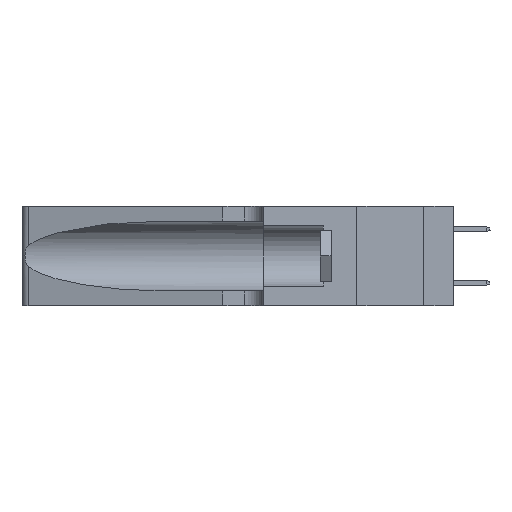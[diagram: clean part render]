
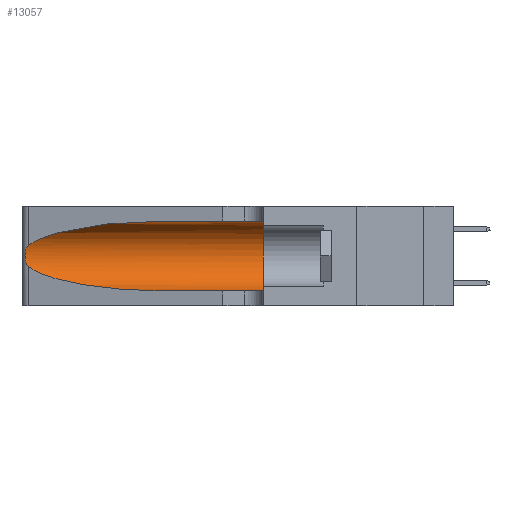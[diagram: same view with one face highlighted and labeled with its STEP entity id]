
A CAD part, left-side view. The second image highlights one B-rep face of the part: STEP entity #13057.
In plain terms, the highlighted cylindrical face has radius 3.308 mm (diameter 6.617 mm), a partial arc.
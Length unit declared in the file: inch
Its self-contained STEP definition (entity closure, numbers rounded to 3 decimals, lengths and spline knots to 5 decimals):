
#863 = ORIENTED_EDGE ( 'NONE', *, *, #18029, .T. ) ;
#1725 = DIRECTION ( 'NONE',  ( 0., 1., 0. ) ) ;
#1914 = CARTESIAN_POINT ( 'NONE',  ( 0.25856, 1.23593, 0.16098 ) ) ;
#2134 = CARTESIAN_POINT ( 'NONE',  ( 0.25555, 1.22994, 0.2215 ) ) ;
#2433 = EDGE_CURVE ( 'NONE', #37462, #30341, #22321, .T. ) ;
#3143 = VERTEX_POINT ( 'NONE', #30191 ) ;
#4962 = AXIS2_PLACEMENT_3D ( 'NONE', #8616, #1725, #5499 ) ;
#5132 = DIRECTION ( 'NONE',  ( 0., 0., -1. ) ) ;
#5239 = CARTESIAN_POINT ( 'NONE',  ( 0.26075, 1.23896, 0.178 ) ) ;
#5499 = DIRECTION ( 'NONE',  ( 0., 0., 1. ) ) ;
#6105 = DIRECTION ( 'NONE',  ( 0., -1., 0. ) ) ;
#6363 = EDGE_CURVE ( 'NONE', #30341, #28219, #10598, .T. ) ;
#8273 = EDGE_CURVE ( 'NONE', #3143, #10191, #37781, .T. ) ;
#8577 = CARTESIAN_POINT ( 'NONE',  ( 0.26018, 1.23835, 0.19895 ) ) ;
#8616 = CARTESIAN_POINT ( 'NONE',  ( 0.1305, 0.35, 0.185 ) ) ;
#9137 = ORIENTED_EDGE ( 'NONE', *, *, #8273, .T. ) ;
#10191 = VERTEX_POINT ( 'NONE', #12703 ) ;
#10598 = CIRCLE ( 'NONE', #4962, 0.13025 ) ;
#10744 = ORIENTED_EDGE ( 'NONE', *, *, #6363, .F. ) ;
#10781 = CARTESIAN_POINT ( 'NONE',  ( 0.18966, 0.96281, 0.31525 ) ) ;
#11106 = FACE_OUTER_BOUND ( 'NONE', #35113, .T. ) ;
#11331 = CYLINDRICAL_SURFACE ( 'NONE', #17786, 0.13025 ) ;
#11534 = CARTESIAN_POINT ( 'NONE',  ( 0.25487, 1.22718, 0.14631 ) ) ;
#12703 = CARTESIAN_POINT ( 'NONE',  ( 0.25487, 1.22718, 0.14631 ) ) ;
#13057 = ADVANCED_FACE ( 'NONE', ( #11106 ), #11331, .F. ) ;
#13968 = CARTESIAN_POINT ( 'NONE',  ( 0.2373, 1.15595, 0.08982 ) ) ;
#14073 = CARTESIAN_POINT ( 'NONE',  ( 0.1305, 0.72297, 0.31525 ) ) ;
#15653 = CARTESIAN_POINT ( 'NONE',  ( 0.25854, 1.2359, 0.20912 ) ) ;
#16092 = CARTESIAN_POINT ( 'NONE',  ( 0.1305, 1.61858, 0.05475 ) ) ;
#16347 = VECTOR ( 'NONE', #6105, 39.37008 ) ;
#17304 =( BOUNDED_CURVE ( )  B_SPLINE_CURVE ( 3, ( #41151, #10781, #40265, #23463 ),
 .UNSPECIFIED., .F., .T. ) 
 B_SPLINE_CURVE_WITH_KNOTS ( ( 4, 4 ),
 ( 1.5708, 2.84003 ),
 .UNSPECIFIED. ) 
 CURVE ( )  GEOMETRIC_REPRESENTATION_ITEM ( )  RATIONAL_B_SPLINE_CURVE ( ( 1., 0.87, 0.87, 1. ) ) 
 REPRESENTATION_ITEM ( '' )  );
#17517 = CARTESIAN_POINT ( 'NONE',  ( 0.1305, 0.72297, 0.05475 ) ) ;
#17786 = AXIS2_PLACEMENT_3D ( 'NONE', #25350, #35471, #5132 ) ;
#18029 = EDGE_CURVE ( 'NONE', #37462, #3143, #17304, .T. ) ;
#18058 = ORIENTED_EDGE ( 'NONE', *, *, #42897, .T. ) ;
#19828 = CARTESIAN_POINT ( 'NONE',  ( 0.25555, 1.22993, 0.14849 ) ) ;
#22021 = VERTEX_POINT ( 'NONE', #35076 ) ;
#22321 = LINE ( 'NONE', #32707, #16347 ) ;
#22568 = DIRECTION ( 'NONE',  ( 0., -1., 0. ) ) ;
#23463 = CARTESIAN_POINT ( 'NONE',  ( 0.25487, 1.22718, 0.22369 ) ) ;
#24613 = ORIENTED_EDGE ( 'NONE', *, *, #37897, .T. ) ;
#25350 = CARTESIAN_POINT ( 'NONE',  ( 0.1305, 1.61858, 0.185 ) ) ;
#25459 = CARTESIAN_POINT ( 'NONE',  ( 0.25639, 1.23184, 0.21858 ) ) ;
#27272 = CARTESIAN_POINT ( 'NONE',  ( 0.1305, 0.35, 0.31525 ) ) ;
#28219 = VERTEX_POINT ( 'NONE', #38660 ) ;
#29186 = CARTESIAN_POINT ( 'NONE',  ( 0.26075, 1.23896, 0.19203 ) ) ;
#30023 = CARTESIAN_POINT ( 'NONE',  ( 0.25487, 1.22718, 0.14631 ) ) ;
#30191 = CARTESIAN_POINT ( 'NONE',  ( 0.25487, 1.22718, 0.22369 ) ) ;
#30242 = CARTESIAN_POINT ( 'NONE',  ( 0.25639, 1.23186, 0.15144 ) ) ;
#30341 = VERTEX_POINT ( 'NONE', #27272 ) ;
#30825 = CARTESIAN_POINT ( 'NONE',  ( 0.18966, 0.96281, 0.05475 ) ) ;
#32271 = CARTESIAN_POINT ( 'NONE',  ( 0.26017, 1.23833, 0.17102 ) ) ;
#32707 = CARTESIAN_POINT ( 'NONE',  ( 0.1305, 1.61858, 0.31525 ) ) ;
#32940 = LINE ( 'NONE', #16092, #36297 ) ;
#35076 = CARTESIAN_POINT ( 'NONE',  ( 0.1305, 0.72297, 0.05475 ) ) ;
#35113 = EDGE_LOOP ( 'NONE', ( #863, #9137, #24613, #18058, #10744, #40123 ) ) ;
#35471 = DIRECTION ( 'NONE',  ( 0., -1., 0. ) ) ;
#35581 = CARTESIAN_POINT ( 'NONE',  ( 0.25487, 1.22718, 0.22369 ) ) ;
#35684 =( BOUNDED_CURVE ( )  B_SPLINE_CURVE ( 3, ( #11534, #13968, #30825, #17517 ),
 .UNSPECIFIED., .F., .T. ) 
 B_SPLINE_CURVE_WITH_KNOTS ( ( 4, 4 ),
 ( 3.44316, 4.71239 ),
 .UNSPECIFIED. ) 
 CURVE ( )  GEOMETRIC_REPRESENTATION_ITEM ( )  RATIONAL_B_SPLINE_CURVE ( ( 1., 0.87, 0.87, 1. ) ) 
 REPRESENTATION_ITEM ( '' )  );
#36297 = VECTOR ( 'NONE', #22568, 39.37008 ) ;
#37462 = VERTEX_POINT ( 'NONE', #14073 ) ;
#37781 = B_SPLINE_CURVE_WITH_KNOTS ( 'NONE', 3,
 ( #35581, #2134, #25459, #38939, #15653, #8577, #29186, #5239, #32271, #1914, #41804, #30242, #19828, #30023 ),
 .UNSPECIFIED., .F., .F.,
 ( 4, 2, 2, 2, 2, 2, 4 ),
 ( 0., 0.00027, 0.00053, 0.00107, 0.0016, 0.00187, 0.00214 ),
 .UNSPECIFIED. ) ;
#37897 = EDGE_CURVE ( 'NONE', #10191, #22021, #35684, .T. ) ;
#38660 = CARTESIAN_POINT ( 'NONE',  ( 0.1305, 0.35, 0.05475 ) ) ;
#38939 = CARTESIAN_POINT ( 'NONE',  ( 0.25787, 1.23484, 0.2124 ) ) ;
#40123 = ORIENTED_EDGE ( 'NONE', *, *, #2433, .F. ) ;
#40265 = CARTESIAN_POINT ( 'NONE',  ( 0.2373, 1.15595, 0.28018 ) ) ;
#41151 = CARTESIAN_POINT ( 'NONE',  ( 0.1305, 0.72297, 0.31525 ) ) ;
#41804 = CARTESIAN_POINT ( 'NONE',  ( 0.25789, 1.23486, 0.15765 ) ) ;
#42897 = EDGE_CURVE ( 'NONE', #22021, #28219, #32940, .T. ) ;
